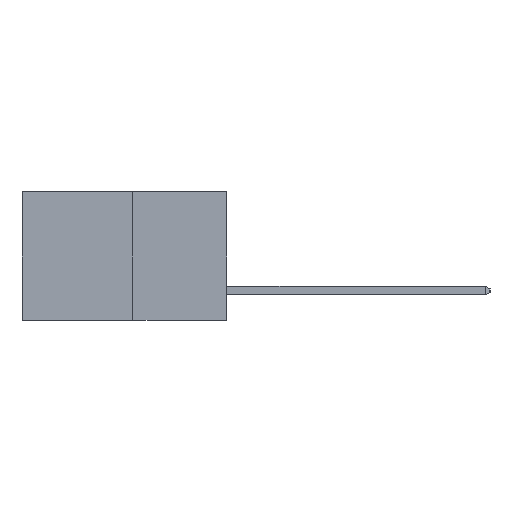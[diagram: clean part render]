
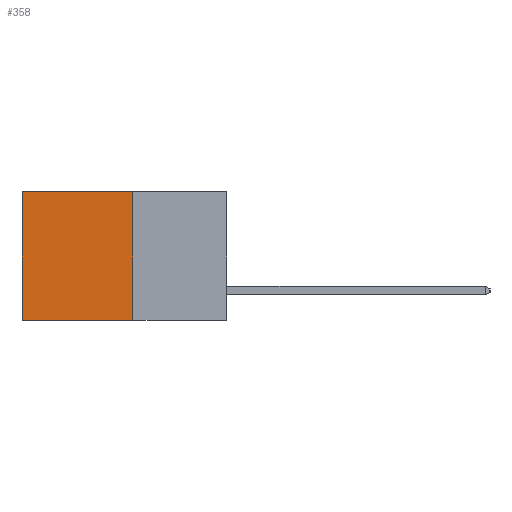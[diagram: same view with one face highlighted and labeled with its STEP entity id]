
A CAD part, left-side view. The second image highlights one B-rep face of the part: STEP entity #358.
In plain terms, the highlighted planar face has unit normal (-1, 0, 0).
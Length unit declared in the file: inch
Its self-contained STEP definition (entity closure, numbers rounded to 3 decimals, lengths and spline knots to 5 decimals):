
#128 = LINE ( 'NONE', #8256, #2586 ) ;
#205 = VERTEX_POINT ( 'NONE', #6274 ) ;
#358 = ADVANCED_FACE ( 'NONE', ( #10868 ), #2700, .F. ) ;
#379 = DIRECTION ( 'NONE',  ( 0., 1., 0. ) ) ;
#438 = ORIENTED_EDGE ( 'NONE', *, *, #4762, .F. ) ;
#1061 = CARTESIAN_POINT ( 'NONE',  ( 0.277, 0.27, 0. ) ) ;
#1197 = ORIENTED_EDGE ( 'NONE', *, *, #1203, .T. ) ;
#1203 = EDGE_CURVE ( 'NONE', #2626, #7409, #10268, .T. ) ;
#1246 = VECTOR ( 'NONE', #10197, 39.37008 ) ;
#1865 = ORIENTED_EDGE ( 'NONE', *, *, #6355, .T. ) ;
#2569 = DIRECTION ( 'NONE',  ( 0., 0., -1. ) ) ;
#2586 = VECTOR ( 'NONE', #3148, 39.37008 ) ;
#2626 = VERTEX_POINT ( 'NONE', #1061 ) ;
#2700 = PLANE ( 'NONE',  #4182 ) ;
#2887 = CARTESIAN_POINT ( 'NONE',  ( 0.277, 0.27, -0.37 ) ) ;
#3148 = DIRECTION ( 'NONE',  ( 0., 1., 0. ) ) ;
#3275 = EDGE_LOOP ( 'NONE', ( #1865, #4946, #438, #1197 ) ) ;
#4182 = AXIS2_PLACEMENT_3D ( 'NONE', #2887, #8759, #6407 ) ;
#4218 = CARTESIAN_POINT ( 'NONE',  ( 0.277, 0.27, -0.37 ) ) ;
#4762 = EDGE_CURVE ( 'NONE', #2626, #205, #8914, .T. ) ;
#4946 = ORIENTED_EDGE ( 'NONE', *, *, #9909, .F. ) ;
#6274 = CARTESIAN_POINT ( 'NONE',  ( 0.277, 0.27, -0.37 ) ) ;
#6355 = EDGE_CURVE ( 'NONE', #7409, #8755, #7888, .T. ) ;
#6407 = DIRECTION ( 'NONE',  ( 0., 0., -1. ) ) ;
#6710 = CARTESIAN_POINT ( 'NONE',  ( 0.277, 0.27, 0. ) ) ;
#6954 = VECTOR ( 'NONE', #2569, 39.37008 ) ;
#7409 = VERTEX_POINT ( 'NONE', #7483 ) ;
#7483 = CARTESIAN_POINT ( 'NONE',  ( 0.277, 0.59, 0. ) ) ;
#7888 = LINE ( 'NONE', #10183, #1246 ) ;
#8243 = VECTOR ( 'NONE', #379, 39.37008 ) ;
#8256 = CARTESIAN_POINT ( 'NONE',  ( 0.277, 0.27, -0.37 ) ) ;
#8755 = VERTEX_POINT ( 'NONE', #9445 ) ;
#8759 = DIRECTION ( 'NONE',  ( 1., 0., 0. ) ) ;
#8914 = LINE ( 'NONE', #4218, #6954 ) ;
#9445 = CARTESIAN_POINT ( 'NONE',  ( 0.277, 0.59, -0.37 ) ) ;
#9909 = EDGE_CURVE ( 'NONE', #205, #8755, #128, .T. ) ;
#10183 = CARTESIAN_POINT ( 'NONE',  ( 0.277, 0.59, -0.37 ) ) ;
#10197 = DIRECTION ( 'NONE',  ( 0., 0., -1. ) ) ;
#10268 = LINE ( 'NONE', #6710, #8243 ) ;
#10868 = FACE_OUTER_BOUND ( 'NONE', #3275, .T. ) ;
